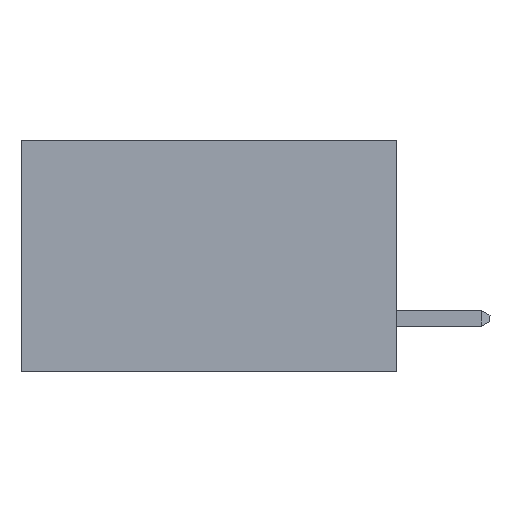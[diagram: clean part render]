
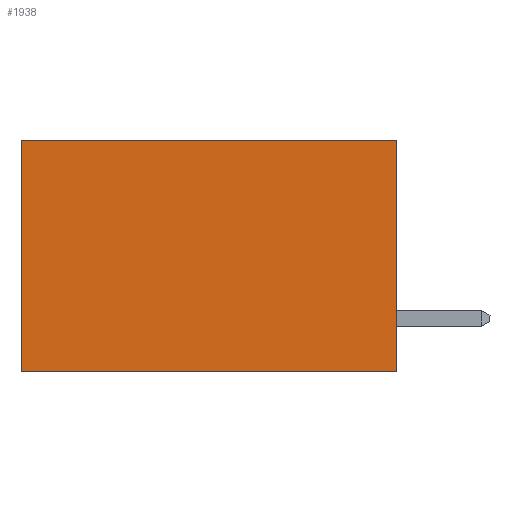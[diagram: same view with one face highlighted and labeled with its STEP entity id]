
A CAD part, left-side view. The second image highlights one B-rep face of the part: STEP entity #1938.
In plain terms, the highlighted planar face has unit normal (-1, 0, 0).
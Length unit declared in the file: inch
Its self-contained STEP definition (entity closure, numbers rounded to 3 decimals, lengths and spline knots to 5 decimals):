
#252 = CARTESIAN_POINT ( 'NONE',  ( 0.2615, 0., 0. ) ) ;
#366 = DIRECTION ( 'NONE',  ( 0., 1., 0. ) ) ;
#685 = CARTESIAN_POINT ( 'NONE',  ( 0.2615, 0.6, -0.37 ) ) ;
#1223 = DIRECTION ( 'NONE',  ( 0., 0., -1. ) ) ;
#1260 = CARTESIAN_POINT ( 'NONE',  ( 0.2615, 0., -0.37 ) ) ;
#1474 = VERTEX_POINT ( 'NONE', #1260 ) ;
#1774 = VECTOR ( 'NONE', #366, 39.37008 ) ;
#1815 = CARTESIAN_POINT ( 'NONE',  ( 0.2615, 0.6, -0.37 ) ) ;
#1835 = LINE ( 'NONE', #5349, #9300 ) ;
#1938 = ADVANCED_FACE ( 'NONE', ( #5461 ), #4821, .F. ) ;
#2262 = LINE ( 'NONE', #252, #1774 ) ;
#3443 = DIRECTION ( 'NONE',  ( 0., 0., -1. ) ) ;
#4046 = EDGE_CURVE ( 'NONE', #5867, #7368, #2262, .T. ) ;
#4548 = DIRECTION ( 'NONE',  ( 0., 0., -1. ) ) ;
#4662 = DIRECTION ( 'NONE',  ( 1., 0., 0. ) ) ;
#4765 = VERTEX_POINT ( 'NONE', #685 ) ;
#4780 = CARTESIAN_POINT ( 'NONE',  ( 0.2615, 0.6, 0. ) ) ;
#4821 = PLANE ( 'NONE',  #9016 ) ;
#4994 = ORIENTED_EDGE ( 'NONE', *, *, #7183, .F. ) ;
#5062 = CARTESIAN_POINT ( 'NONE',  ( 0.2615, 0., -0.37 ) ) ;
#5066 = EDGE_CURVE ( 'NONE', #7368, #4765, #9024, .T. ) ;
#5183 = EDGE_LOOP ( 'NONE', ( #5968, #4994, #6089, #5659 ) ) ;
#5349 = CARTESIAN_POINT ( 'NONE',  ( 0.2615, 0., -0.37 ) ) ;
#5461 = FACE_OUTER_BOUND ( 'NONE', #5183, .T. ) ;
#5659 = ORIENTED_EDGE ( 'NONE', *, *, #4046, .T. ) ;
#5784 = CARTESIAN_POINT ( 'NONE',  ( 0.2615, 0., -0.37 ) ) ;
#5867 = VERTEX_POINT ( 'NONE', #9032 ) ;
#5968 = ORIENTED_EDGE ( 'NONE', *, *, #5066, .T. ) ;
#6056 = DIRECTION ( 'NONE',  ( 0., 1., 0. ) ) ;
#6089 = ORIENTED_EDGE ( 'NONE', *, *, #6861, .F. ) ;
#6390 = LINE ( 'NONE', #5784, #8464 ) ;
#6861 = EDGE_CURVE ( 'NONE', #5867, #1474, #6390, .T. ) ;
#7183 = EDGE_CURVE ( 'NONE', #1474, #4765, #1835, .T. ) ;
#7196 = VECTOR ( 'NONE', #3443, 39.37008 ) ;
#7368 = VERTEX_POINT ( 'NONE', #4780 ) ;
#8464 = VECTOR ( 'NONE', #1223, 39.37008 ) ;
#9016 = AXIS2_PLACEMENT_3D ( 'NONE', #5062, #4662, #4548 ) ;
#9024 = LINE ( 'NONE', #1815, #7196 ) ;
#9032 = CARTESIAN_POINT ( 'NONE',  ( 0.2615, 0., 0. ) ) ;
#9300 = VECTOR ( 'NONE', #6056, 39.37008 ) ;
